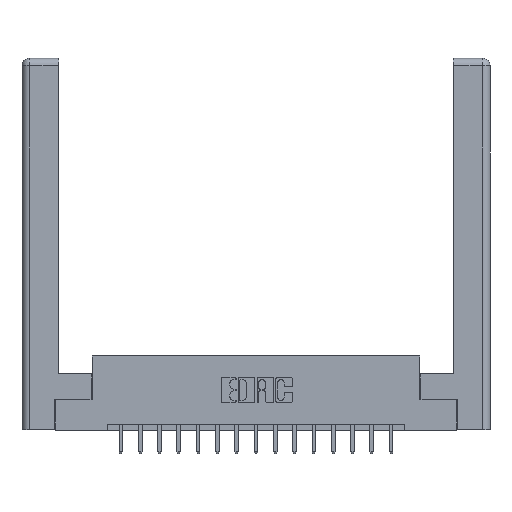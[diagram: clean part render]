
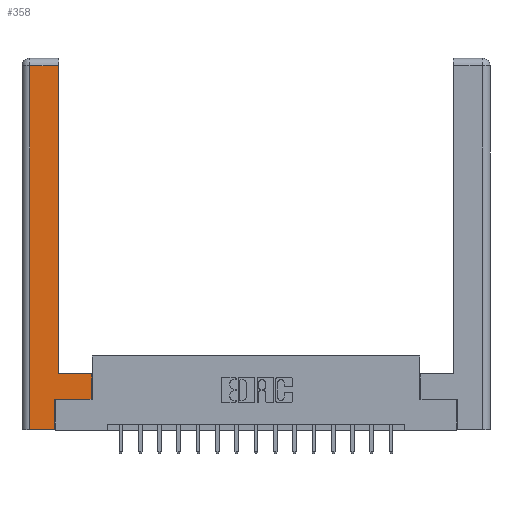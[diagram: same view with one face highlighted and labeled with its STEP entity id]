
A CAD part, top view. The second image highlights one B-rep face of the part: STEP entity #358.
In plain terms, the highlighted planar face has unit normal (0, 0, 1).
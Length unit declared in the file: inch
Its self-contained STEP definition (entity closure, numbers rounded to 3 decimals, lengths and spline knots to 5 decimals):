
#241 = VECTOR ( 'NONE', #6637, 39.37008 ) ;
#271 = ORIENTED_EDGE ( 'NONE', *, *, #15866, .T. ) ;
#358 = ADVANCED_FACE ( 'NONE', ( #15851 ), #11609, .F. ) ;
#369 = VERTEX_POINT ( 'NONE', #1825 ) ;
#570 = VECTOR ( 'NONE', #10417, 39.37008 ) ;
#690 = CARTESIAN_POINT ( 'NONE',  ( 0.295, 0.45, 0. ) ) ;
#969 = EDGE_CURVE ( 'NONE', #10719, #369, #13640, .T. ) ;
#1039 = VECTOR ( 'NONE', #1494, 39.37008 ) ;
#1162 = VECTOR ( 'NONE', #2404, 39.37008 ) ;
#1373 = VERTEX_POINT ( 'NONE', #690 ) ;
#1494 = DIRECTION ( 'NONE',  ( 0., 1., 0. ) ) ;
#1674 = EDGE_CURVE ( 'NONE', #12384, #4931, #6716, .T. ) ;
#1825 = CARTESIAN_POINT ( 'NONE',  ( 0.565, 0.45, 0. ) ) ;
#2360 = EDGE_CURVE ( 'NONE', #5196, #12384, #6682, .T. ) ;
#2404 = DIRECTION ( 'NONE',  ( 0., 1., 0. ) ) ;
#3078 = DIRECTION ( 'NONE',  ( -1., 0., 0. ) ) ;
#3106 = CARTESIAN_POINT ( 'NONE',  ( 0.265, 0.245, 0. ) ) ;
#3201 = ORIENTED_EDGE ( 'NONE', *, *, #4790, .T. ) ;
#3245 = CARTESIAN_POINT ( 'NONE',  ( 0.265, 0.245, 0. ) ) ;
#3317 = LINE ( 'NONE', #10051, #13901 ) ;
#3478 = AXIS2_PLACEMENT_3D ( 'NONE', #11349, #15614, #3078 ) ;
#4060 = ORIENTED_EDGE ( 'NONE', *, *, #969, .T. ) ;
#4201 = VECTOR ( 'NONE', #14614, 39.37008 ) ;
#4790 = EDGE_CURVE ( 'NONE', #369, #1373, #14199, .T. ) ;
#4931 = VERTEX_POINT ( 'NONE', #8538 ) ;
#5196 = VERTEX_POINT ( 'NONE', #10039 ) ;
#5728 = ORIENTED_EDGE ( 'NONE', *, *, #14868, .T. ) ;
#6637 = DIRECTION ( 'NONE',  ( 0., -1., 0. ) ) ;
#6682 = LINE ( 'NONE', #16435, #15361 ) ;
#6716 = LINE ( 'NONE', #6757, #241 ) ;
#6757 = CARTESIAN_POINT ( 'NONE',  ( 0.0615, 0., 0. ) ) ;
#6789 = DIRECTION ( 'NONE',  ( -1., 0., 0. ) ) ;
#7071 = ORIENTED_EDGE ( 'NONE', *, *, #1674, .T. ) ;
#7166 = CARTESIAN_POINT ( 'NONE',  ( 0.0615, 2.94, 0. ) ) ;
#7187 = EDGE_LOOP ( 'NONE', ( #17625, #7407, #7071, #5728, #10627, #271, #4060, #3201 ) ) ;
#7407 = ORIENTED_EDGE ( 'NONE', *, *, #2360, .T. ) ;
#8177 = VERTEX_POINT ( 'NONE', #10836 ) ;
#8538 = CARTESIAN_POINT ( 'NONE',  ( 0.0615, 0., 0. ) ) ;
#8661 = VECTOR ( 'NONE', #15328, 39.37008 ) ;
#8920 = LINE ( 'NONE', #10661, #1162 ) ;
#10039 = CARTESIAN_POINT ( 'NONE',  ( 0.295, 2.94, 0. ) ) ;
#10051 = CARTESIAN_POINT ( 'NONE',  ( 0.565, 0.245, 0. ) ) ;
#10394 = CARTESIAN_POINT ( 'NONE',  ( 0.565, 0.245, 0. ) ) ;
#10417 = DIRECTION ( 'NONE',  ( -1., 0., 0. ) ) ;
#10627 = ORIENTED_EDGE ( 'NONE', *, *, #12380, .T. ) ;
#10661 = CARTESIAN_POINT ( 'NONE',  ( 0.295, 3., 0. ) ) ;
#10719 = VERTEX_POINT ( 'NONE', #10394 ) ;
#10836 = CARTESIAN_POINT ( 'NONE',  ( 0.265, 0., 0. ) ) ;
#11349 = CARTESIAN_POINT ( 'NONE',  ( 0., 0., 0. ) ) ;
#11609 = PLANE ( 'NONE',  #3478 ) ;
#12047 = LINE ( 'NONE', #3106, #1039 ) ;
#12380 = EDGE_CURVE ( 'NONE', #8177, #12910, #12047, .T. ) ;
#12384 = VERTEX_POINT ( 'NONE', #7166 ) ;
#12910 = VERTEX_POINT ( 'NONE', #3245 ) ;
#13640 = LINE ( 'NONE', #17042, #8661 ) ;
#13901 = VECTOR ( 'NONE', #14130, 39.37008 ) ;
#14130 = DIRECTION ( 'NONE',  ( 1., 0., 0. ) ) ;
#14199 = LINE ( 'NONE', #17327, #570 ) ;
#14614 = DIRECTION ( 'NONE',  ( 1., 0., 0. ) ) ;
#14868 = EDGE_CURVE ( 'NONE', #4931, #8177, #16333, .T. ) ;
#15328 = DIRECTION ( 'NONE',  ( 0., 1., 0. ) ) ;
#15361 = VECTOR ( 'NONE', #6789, 39.37008 ) ;
#15600 = EDGE_CURVE ( 'NONE', #1373, #5196, #8920, .T. ) ;
#15614 = DIRECTION ( 'NONE',  ( 0., 0., -1. ) ) ;
#15851 = FACE_OUTER_BOUND ( 'NONE', #7187, .T. ) ;
#15866 = EDGE_CURVE ( 'NONE', #12910, #10719, #3317, .T. ) ;
#16333 = LINE ( 'NONE', #17317, #4201 ) ;
#16435 = CARTESIAN_POINT ( 'NONE',  ( 0.0615, 2.94, 0. ) ) ;
#17042 = CARTESIAN_POINT ( 'NONE',  ( 0.565, 0.45, 0. ) ) ;
#17317 = CARTESIAN_POINT ( 'NONE',  ( 0.265, 0., 0. ) ) ;
#17327 = CARTESIAN_POINT ( 'NONE',  ( 0.295, 0.45, 0. ) ) ;
#17625 = ORIENTED_EDGE ( 'NONE', *, *, #15600, .T. ) ;
